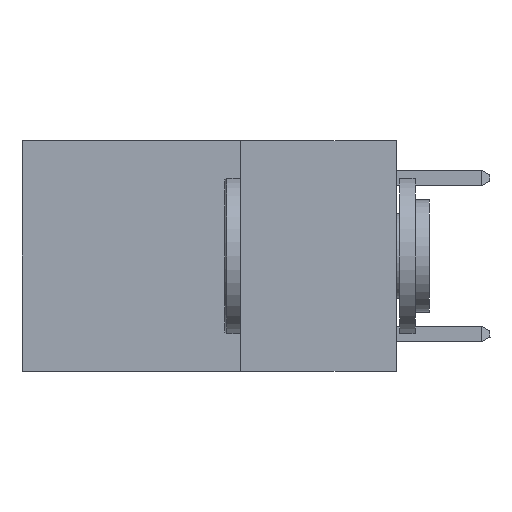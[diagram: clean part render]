
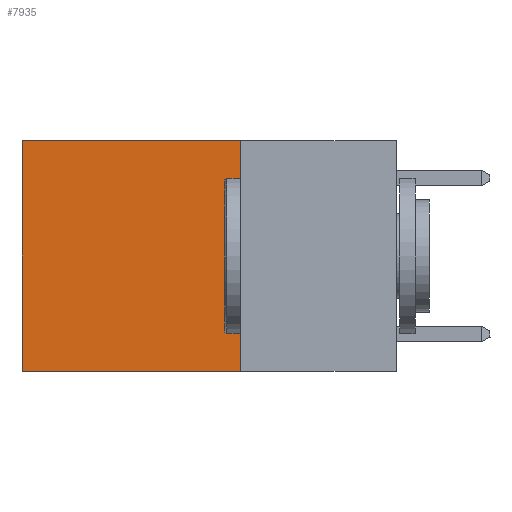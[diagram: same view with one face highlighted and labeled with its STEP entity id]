
A CAD part, left-side view. The second image highlights one B-rep face of the part: STEP entity #7935.
In plain terms, the highlighted planar face has unit normal (-1, 0, 0).
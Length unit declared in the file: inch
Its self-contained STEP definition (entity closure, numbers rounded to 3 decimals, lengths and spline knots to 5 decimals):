
#689 = LINE ( 'NONE', #19569, #964 ) ;
#964 = VECTOR ( 'NONE', #25273, 39.37008 ) ;
#3725 = CARTESIAN_POINT ( 'NONE',  ( 0.2625, 0.6, 0. ) ) ;
#3887 = FACE_OUTER_BOUND ( 'NONE', #23789, .T. ) ;
#4902 = CARTESIAN_POINT ( 'NONE',  ( 0.2625, 0.25, 0. ) ) ;
#5000 = DIRECTION ( 'NONE',  ( 0., 0., -1. ) ) ;
#5015 = DIRECTION ( 'NONE',  ( 0., 0., -1. ) ) ;
#5715 = ORIENTED_EDGE ( 'NONE', *, *, #10647, .T. ) ;
#5845 = VECTOR ( 'NONE', #11132, 39.37008 ) ;
#5995 = LINE ( 'NONE', #4902, #5845 ) ;
#7935 = ADVANCED_FACE ( 'NONE', ( #3887 ), #15205, .F. ) ;
#9199 = VERTEX_POINT ( 'NONE', #14845 ) ;
#9219 = ORIENTED_EDGE ( 'NONE', *, *, #13418, .F. ) ;
#10615 = VECTOR ( 'NONE', #5015, 39.37008 ) ;
#10647 = EDGE_CURVE ( 'NONE', #12523, #21672, #10765, .T. ) ;
#10765 = LINE ( 'NONE', #15134, #10615 ) ;
#11040 = CARTESIAN_POINT ( 'NONE',  ( 0.2625, 0.25, 0. ) ) ;
#11132 = DIRECTION ( 'NONE',  ( 0., 1., 0. ) ) ;
#12425 = VECTOR ( 'NONE', #22964, 39.37008 ) ;
#12523 = VERTEX_POINT ( 'NONE', #3725 ) ;
#12574 = LINE ( 'NONE', #21014, #12425 ) ;
#13418 = EDGE_CURVE ( 'NONE', #15940, #9199, #12574, .T. ) ;
#14047 = CARTESIAN_POINT ( 'NONE',  ( 0.2625, 0.25, 0. ) ) ;
#14384 = EDGE_CURVE ( 'NONE', #15940, #12523, #5995, .T. ) ;
#14845 = CARTESIAN_POINT ( 'NONE',  ( 0.2625, 0.25, -0.37 ) ) ;
#15097 = EDGE_CURVE ( 'NONE', #9199, #21672, #689, .T. ) ;
#15134 = CARTESIAN_POINT ( 'NONE',  ( 0.2625, 0.6, 0. ) ) ;
#15205 = PLANE ( 'NONE',  #24346 ) ;
#15940 = VERTEX_POINT ( 'NONE', #14047 ) ;
#16461 = CARTESIAN_POINT ( 'NONE',  ( 0.2625, 0.6, -0.37 ) ) ;
#17260 = DIRECTION ( 'NONE',  ( 1., 0., 0. ) ) ;
#18646 = ORIENTED_EDGE ( 'NONE', *, *, #14384, .T. ) ;
#19569 = CARTESIAN_POINT ( 'NONE',  ( 0.2625, 0.25, -0.37 ) ) ;
#21014 = CARTESIAN_POINT ( 'NONE',  ( 0.2625, 0.25, 0. ) ) ;
#21672 = VERTEX_POINT ( 'NONE', #16461 ) ;
#22688 = ORIENTED_EDGE ( 'NONE', *, *, #15097, .F. ) ;
#22964 = DIRECTION ( 'NONE',  ( 0., 0., -1. ) ) ;
#23789 = EDGE_LOOP ( 'NONE', ( #5715, #22688, #9219, #18646 ) ) ;
#24346 = AXIS2_PLACEMENT_3D ( 'NONE', #11040, #17260, #5000 ) ;
#25273 = DIRECTION ( 'NONE',  ( 0., 1., 0. ) ) ;
